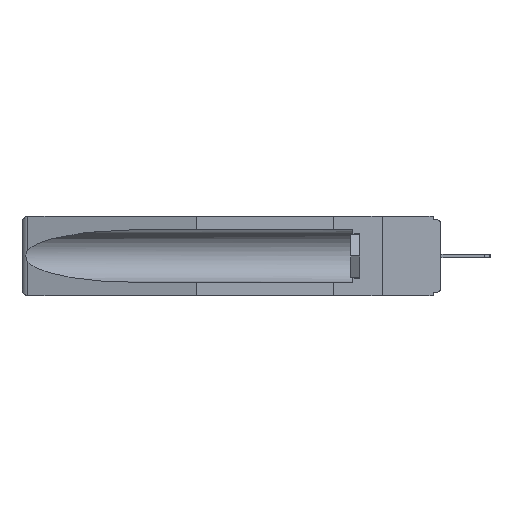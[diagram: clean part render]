
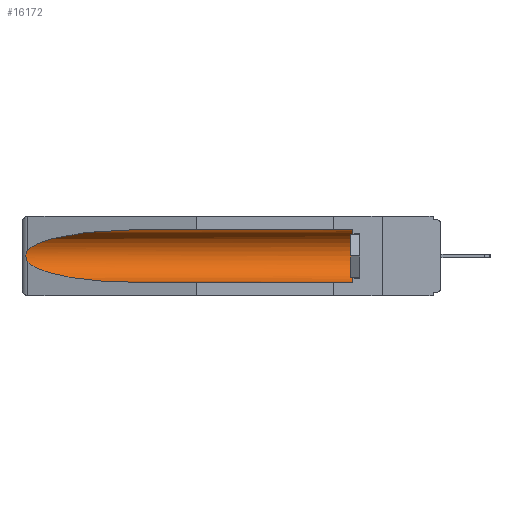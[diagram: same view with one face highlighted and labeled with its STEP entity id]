
A CAD part, left-side view. The second image highlights one B-rep face of the part: STEP entity #16172.
In plain terms, the highlighted cylindrical face has radius 2.857 mm (diameter 5.715 mm), a partial arc.
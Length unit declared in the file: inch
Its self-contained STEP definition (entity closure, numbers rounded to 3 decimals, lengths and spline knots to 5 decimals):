
#203 = DIRECTION ( 'NONE',  ( 0., 0., 1. ) ) ;
#308 = VERTEX_POINT ( 'NONE', #18713 ) ;
#326 = CARTESIAN_POINT ( 'NONE',  ( 0.26537, 1.52718, -0.19328 ) ) ;
#523 = CIRCLE ( 'NONE', #11711, 0.1125 ) ;
#876 = VECTOR ( 'NONE', #12404, 39.37008 ) ;
#1395 = CYLINDRICAL_SURFACE ( 'NONE', #19333, 0.1125 ) ;
#3263 = ORIENTED_EDGE ( 'NONE', *, *, #24766, .T. ) ;
#3314 = LINE ( 'NONE', #13461, #24815 ) ;
#3331 = DIRECTION ( 'NONE',  ( 0., 1., 0. ) ) ;
#3767 = ORIENTED_EDGE ( 'NONE', *, *, #12577, .T. ) ;
#3969 = CARTESIAN_POINT ( 'NONE',  ( 0.155, -0.30754, -0.059 ) ) ;
#4886 = EDGE_LOOP ( 'NONE', ( #23007, #3767, #12959, #15667, #3263, #26233 ) ) ;
#5290 = VERTEX_POINT ( 'NONE', #6268 ) ;
#5507 = DIRECTION ( 'NONE',  ( 0., 0., 1. ) ) ;
#5948 = CARTESIAN_POINT ( 'NONE',  ( 0.26537, 1.52718, -0.14972 ) ) ;
#6093 = VERTEX_POINT ( 'NONE', #25518 ) ;
#6268 = CARTESIAN_POINT ( 'NONE',  ( 0.155, 0.126, -0.059 ) ) ;
#6731 = EDGE_CURVE ( 'NONE', #308, #6093, #3314, .T. ) ;
#6754 = CARTESIAN_POINT ( 'NONE',  ( 0.155, 1.07973, -0.059 ) ) ;
#6838 = CARTESIAN_POINT ( 'NONE',  ( 0.21114, 1.30732, -0.284 ) ) ;
#7128 = FACE_OUTER_BOUND ( 'NONE', #4886, .T. ) ;
#8062 = CARTESIAN_POINT ( 'NONE',  ( 0.2675, 1.53308, -0.16763 ) ) ;
#8353 = CARTESIAN_POINT ( 'NONE',  ( 0.26537, 1.52718, -0.19328 ) ) ;
#8743 =( BOUNDED_CURVE ( )  B_SPLINE_CURVE ( 3, ( #326, #13098, #6838, #21337 ),
 .UNSPECIFIED., .F., .F. ) 
 B_SPLINE_CURVE_WITH_KNOTS ( ( 4, 4 ),
 ( 0.1948, 1.5708 ),
 .UNSPECIFIED. ) 
 CURVE ( )  GEOMETRIC_REPRESENTATION_ITEM ( )  RATIONAL_B_SPLINE_CURVE ( ( 1., 0.848, 0.848, 1. ) ) 
 REPRESENTATION_ITEM ( '' )  );
#10127 = CARTESIAN_POINT ( 'NONE',  ( 0.26597, 1.52961, -0.15275 ) ) ;
#10210 = CARTESIAN_POINT ( 'NONE',  ( 0.2673, 1.53269, -0.17917 ) ) ;
#10608 = B_SPLINE_CURVE_WITH_KNOTS ( 'NONE', 3,
 ( #5948, #10127, #14295, #20468, #8062, #22537, #10210, #24608, #12299, #26692 ),
 .UNSPECIFIED., .F., .F.,
 ( 4, 2, 2, 2, 4 ),
 ( 0., 0.00029, 0.00058, 0.00087, 0.00117 ),
 .UNSPECIFIED. ) ;
#11386 = DIRECTION ( 'NONE',  ( 0., 1., 0. ) ) ;
#11711 = AXIS2_PLACEMENT_3D ( 'NONE', #25275, #12978, #203 ) ;
#12299 = CARTESIAN_POINT ( 'NONE',  ( 0.26597, 1.5296, -0.19026 ) ) ;
#12404 = DIRECTION ( 'NONE',  ( 0., 1., 0. ) ) ;
#12577 = EDGE_CURVE ( 'NONE', #18267, #14645, #10608, .T. ) ;
#12959 = ORIENTED_EDGE ( 'NONE', *, *, #20260, .T. ) ;
#12978 = DIRECTION ( 'NONE',  ( 0., -1., 0. ) ) ;
#13018 = CARTESIAN_POINT ( 'NONE',  ( 0.21114, 1.30732, -0.059 ) ) ;
#13098 = CARTESIAN_POINT ( 'NONE',  ( 0.25451, 1.48313, -0.24835 ) ) ;
#13103 = CARTESIAN_POINT ( 'NONE',  ( 0.26537, 1.52718, -0.14972 ) ) ;
#13461 = CARTESIAN_POINT ( 'NONE',  ( 0.155, -0.30754, -0.284 ) ) ;
#13782 = CARTESIAN_POINT ( 'NONE',  ( 0.155, 1.07973, -0.059 ) ) ;
#14295 = CARTESIAN_POINT ( 'NONE',  ( 0.26654, 1.53092, -0.15636 ) ) ;
#14645 = VERTEX_POINT ( 'NONE', #8353 ) ;
#15667 = ORIENTED_EDGE ( 'NONE', *, *, #6731, .F. ) ;
#16172 = ADVANCED_FACE ( 'NONE', ( #7128 ), #1395, .F. ) ;
#17240 =( BOUNDED_CURVE ( )  B_SPLINE_CURVE ( 3, ( #6754, #13018, #25397, #13103 ),
 .UNSPECIFIED., .F., .F. ) 
 B_SPLINE_CURVE_WITH_KNOTS ( ( 4, 4 ),
 ( 4.71239, 6.08839 ),
 .UNSPECIFIED. ) 
 CURVE ( )  GEOMETRIC_REPRESENTATION_ITEM ( )  RATIONAL_B_SPLINE_CURVE ( ( 1., 0.848, 0.848, 1. ) ) 
 REPRESENTATION_ITEM ( '' )  );
#17920 = CARTESIAN_POINT ( 'NONE',  ( 0.155, -0.30754, -0.1715 ) ) ;
#18267 = VERTEX_POINT ( 'NONE', #20117 ) ;
#18713 = CARTESIAN_POINT ( 'NONE',  ( 0.155, 0.126, -0.284 ) ) ;
#19333 = AXIS2_PLACEMENT_3D ( 'NONE', #17920, #3331, #5507 ) ;
#20117 = CARTESIAN_POINT ( 'NONE',  ( 0.26537, 1.52718, -0.14972 ) ) ;
#20260 = EDGE_CURVE ( 'NONE', #14645, #6093, #8743, .T. ) ;
#20468 = CARTESIAN_POINT ( 'NONE',  ( 0.2673, 1.5327, -0.16383 ) ) ;
#21337 = CARTESIAN_POINT ( 'NONE',  ( 0.155, 1.07973, -0.284 ) ) ;
#22025 = EDGE_CURVE ( 'NONE', #26681, #18267, #17240, .T. ) ;
#22493 = LINE ( 'NONE', #3969, #876 ) ;
#22537 = CARTESIAN_POINT ( 'NONE',  ( 0.2675, 1.53308, -0.17534 ) ) ;
#23007 = ORIENTED_EDGE ( 'NONE', *, *, #22025, .T. ) ;
#24608 = CARTESIAN_POINT ( 'NONE',  ( 0.26655, 1.53094, -0.18657 ) ) ;
#24766 = EDGE_CURVE ( 'NONE', #308, #5290, #523, .T. ) ;
#24815 = VECTOR ( 'NONE', #11386, 39.37008 ) ;
#25211 = EDGE_CURVE ( 'NONE', #5290, #26681, #22493, .T. ) ;
#25275 = CARTESIAN_POINT ( 'NONE',  ( 0.155, 0.126, -0.1715 ) ) ;
#25397 = CARTESIAN_POINT ( 'NONE',  ( 0.25451, 1.48313, -0.09465 ) ) ;
#25518 = CARTESIAN_POINT ( 'NONE',  ( 0.155, 1.07973, -0.284 ) ) ;
#26233 = ORIENTED_EDGE ( 'NONE', *, *, #25211, .T. ) ;
#26681 = VERTEX_POINT ( 'NONE', #13782 ) ;
#26692 = CARTESIAN_POINT ( 'NONE',  ( 0.26537, 1.52718, -0.19328 ) ) ;
